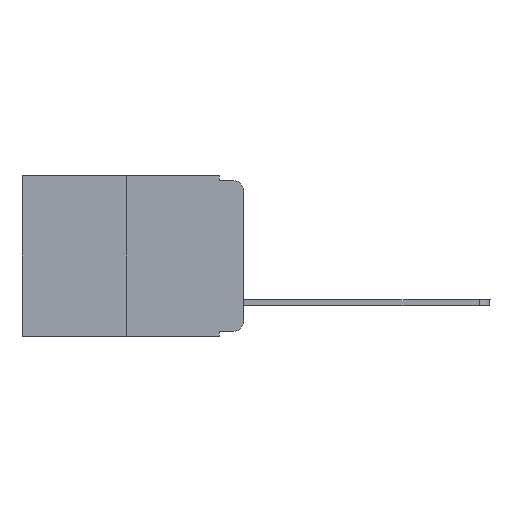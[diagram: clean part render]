
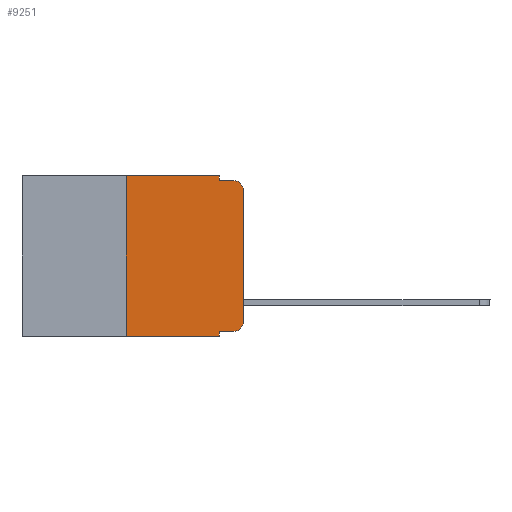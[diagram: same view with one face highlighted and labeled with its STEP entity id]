
A CAD part, left-side view. The second image highlights one B-rep face of the part: STEP entity #9251.
In plain terms, the highlighted planar face has unit normal (-1, 0, 0).
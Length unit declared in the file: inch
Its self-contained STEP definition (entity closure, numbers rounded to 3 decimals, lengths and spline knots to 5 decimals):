
#179 = ORIENTED_EDGE ( 'NONE', *, *, #10352, .F. ) ;
#988 = EDGE_CURVE ( 'NONE', #8281, #11301, #16876, .T. ) ;
#1937 = DIRECTION ( 'NONE',  ( 0., -1., 0. ) ) ;
#2013 = VECTOR ( 'NONE', #4165, 39.37008 ) ;
#2155 = EDGE_CURVE ( 'NONE', #15813, #8210, #14939, .T. ) ;
#2252 = DIRECTION ( 'NONE',  ( 1., 0., 0. ) ) ;
#2440 = ORIENTED_EDGE ( 'NONE', *, *, #14487, .T. ) ;
#2833 = AXIS2_PLACEMENT_3D ( 'NONE', #11135, #2252, #16352 ) ;
#3005 = CARTESIAN_POINT ( 'NONE',  ( 0., 0.25, -0.343 ) ) ;
#3064 = ORIENTED_EDGE ( 'NONE', *, *, #2155, .F. ) ;
#3278 = CARTESIAN_POINT ( 'NONE',  ( 0., 0., -0.313 ) ) ;
#3292 = DIRECTION ( 'NONE',  ( 0., 0., -1. ) ) ;
#3900 = CARTESIAN_POINT ( 'NONE',  ( 0., 0.25, 0. ) ) ;
#4133 = VERTEX_POINT ( 'NONE', #3278 ) ;
#4148 = VECTOR ( 'NONE', #15728, 39.37008 ) ;
#4165 = DIRECTION ( 'NONE',  ( 0., 0., 1. ) ) ;
#4544 = DIRECTION ( 'NONE',  ( 0., -1., 0. ) ) ;
#4918 = LINE ( 'NONE', #11152, #4987 ) ;
#4987 = VECTOR ( 'NONE', #13888, 39.37008 ) ;
#4988 = VERTEX_POINT ( 'NONE', #12117 ) ;
#5269 = VERTEX_POINT ( 'NONE', #10535 ) ;
#5349 = VECTOR ( 'NONE', #11831, 39.37008 ) ;
#5590 = EDGE_CURVE ( 'NONE', #16306, #12319, #11303, .T. ) ;
#5683 = LINE ( 'NONE', #14824, #2013 ) ;
#5846 = CARTESIAN_POINT ( 'NONE',  ( 0., 0.02, -0.313 ) ) ;
#5892 = CARTESIAN_POINT ( 'NONE',  ( 0., 0.051, -0.01 ) ) ;
#5916 = CARTESIAN_POINT ( 'NONE',  ( 0., 0.051, -0.01 ) ) ;
#6602 = EDGE_CURVE ( 'NONE', #11301, #15766, #13377, .T. ) ;
#6634 = LINE ( 'NONE', #9210, #16507 ) ;
#6701 = EDGE_CURVE ( 'NONE', #16306, #5269, #4918, .T. ) ;
#6936 = CARTESIAN_POINT ( 'NONE',  ( 0., 0.02, -0.01 ) ) ;
#7003 = EDGE_LOOP ( 'NONE', ( #9979, #16259, #3064, #179, #8290, #15225, #2440, #8655, #11409, #12706 ) ) ;
#7033 = LINE ( 'NONE', #12232, #15679 ) ;
#7353 = EDGE_CURVE ( 'NONE', #4133, #4988, #5683, .T. ) ;
#7595 = VECTOR ( 'NONE', #4544, 39.37008 ) ;
#8210 = VERTEX_POINT ( 'NONE', #6936 ) ;
#8281 = VERTEX_POINT ( 'NONE', #3005 ) ;
#8290 = ORIENTED_EDGE ( 'NONE', *, *, #6602, .F. ) ;
#8435 = CARTESIAN_POINT ( 'NONE',  ( 0., 0.473, 0. ) ) ;
#8655 = ORIENTED_EDGE ( 'NONE', *, *, #5590, .F. ) ;
#9210 = CARTESIAN_POINT ( 'NONE',  ( 0., 0.051, 0. ) ) ;
#9251 = ADVANCED_FACE ( 'NONE', ( #13693 ), #15228, .F. ) ;
#9775 = DIRECTION ( 'NONE',  ( -1., 0., 0. ) ) ;
#9878 = CIRCLE ( 'NONE', #10936, 0.02 ) ;
#9979 = ORIENTED_EDGE ( 'NONE', *, *, #7353, .T. ) ;
#10352 = EDGE_CURVE ( 'NONE', #15766, #15813, #6634, .T. ) ;
#10412 = VECTOR ( 'NONE', #1937, 39.37008 ) ;
#10535 = CARTESIAN_POINT ( 'NONE',  ( 0., 0.02, -0.333 ) ) ;
#10936 = AXIS2_PLACEMENT_3D ( 'NONE', #5846, #9775, #3292 ) ;
#11135 = CARTESIAN_POINT ( 'NONE',  ( 0., 0.473, 0. ) ) ;
#11142 = DIRECTION ( 'NONE',  ( 0., 0., -1. ) ) ;
#11152 = CARTESIAN_POINT ( 'NONE',  ( 0., 0.051, -0.333 ) ) ;
#11301 = VERTEX_POINT ( 'NONE', #3900 ) ;
#11303 = LINE ( 'NONE', #13259, #4148 ) ;
#11409 = ORIENTED_EDGE ( 'NONE', *, *, #6701, .T. ) ;
#11684 = EDGE_CURVE ( 'NONE', #5269, #4133, #9878, .T. ) ;
#11831 = DIRECTION ( 'NONE',  ( 0., 0., 1. ) ) ;
#11861 = DIRECTION ( 'NONE',  ( 0., 0., -1. ) ) ;
#12117 = CARTESIAN_POINT ( 'NONE',  ( 0., 0., -0.03 ) ) ;
#12232 = CARTESIAN_POINT ( 'NONE',  ( 0., 0.473, -0.343 ) ) ;
#12269 = CARTESIAN_POINT ( 'NONE',  ( 0., 0.051, -0.343 ) ) ;
#12319 = VERTEX_POINT ( 'NONE', #12269 ) ;
#12706 = ORIENTED_EDGE ( 'NONE', *, *, #11684, .T. ) ;
#13047 = CARTESIAN_POINT ( 'NONE',  ( 0., 0.051, -0.333 ) ) ;
#13259 = CARTESIAN_POINT ( 'NONE',  ( 0., 0.051, 0. ) ) ;
#13377 = LINE ( 'NONE', #8435, #10412 ) ;
#13693 = FACE_OUTER_BOUND ( 'NONE', #7003, .T. ) ;
#13746 = AXIS2_PLACEMENT_3D ( 'NONE', #15319, #16437, #11142 ) ;
#13888 = DIRECTION ( 'NONE',  ( 0., -1., 0. ) ) ;
#14461 = CARTESIAN_POINT ( 'NONE',  ( 0., 0.25, 0. ) ) ;
#14487 = EDGE_CURVE ( 'NONE', #8281, #12319, #7033, .T. ) ;
#14824 = CARTESIAN_POINT ( 'NONE',  ( 0., 0., 0. ) ) ;
#14939 = LINE ( 'NONE', #5892, #7595 ) ;
#15225 = ORIENTED_EDGE ( 'NONE', *, *, #988, .F. ) ;
#15228 = PLANE ( 'NONE',  #2833 ) ;
#15319 = CARTESIAN_POINT ( 'NONE',  ( 0., 0.02, -0.03 ) ) ;
#15323 = EDGE_CURVE ( 'NONE', #4988, #8210, #15386, .T. ) ;
#15386 = CIRCLE ( 'NONE', #13746, 0.02 ) ;
#15679 = VECTOR ( 'NONE', #15990, 39.37008 ) ;
#15728 = DIRECTION ( 'NONE',  ( 0., 0., -1. ) ) ;
#15766 = VERTEX_POINT ( 'NONE', #16416 ) ;
#15813 = VERTEX_POINT ( 'NONE', #5916 ) ;
#15990 = DIRECTION ( 'NONE',  ( 0., -1., 0. ) ) ;
#16259 = ORIENTED_EDGE ( 'NONE', *, *, #15323, .T. ) ;
#16306 = VERTEX_POINT ( 'NONE', #13047 ) ;
#16352 = DIRECTION ( 'NONE',  ( 0., 0., -1. ) ) ;
#16416 = CARTESIAN_POINT ( 'NONE',  ( 0., 0.051, 0. ) ) ;
#16437 = DIRECTION ( 'NONE',  ( -1., 0., 0. ) ) ;
#16507 = VECTOR ( 'NONE', #11861, 39.37008 ) ;
#16876 = LINE ( 'NONE', #14461, #5349 ) ;
